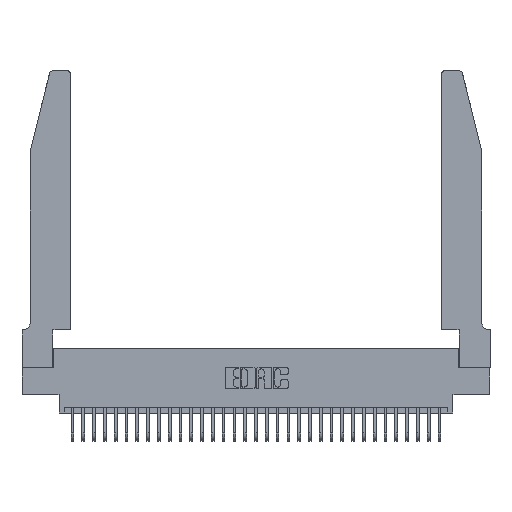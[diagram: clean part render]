
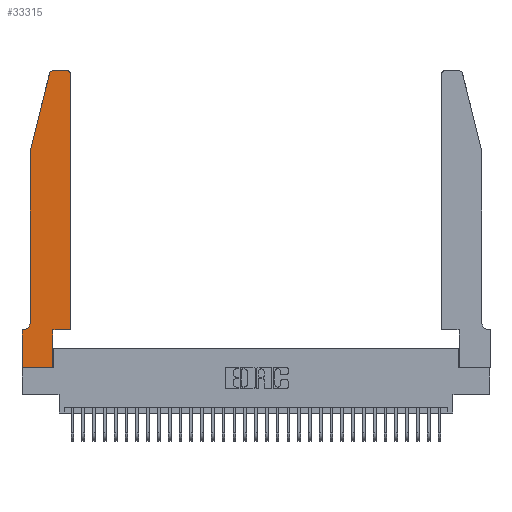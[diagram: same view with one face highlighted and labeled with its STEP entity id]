
A CAD part, top view. The second image highlights one B-rep face of the part: STEP entity #33315.
In plain terms, the highlighted planar face has unit normal (0, 0, 1).
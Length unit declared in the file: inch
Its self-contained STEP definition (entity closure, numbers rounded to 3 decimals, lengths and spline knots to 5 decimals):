
#8 = DIRECTION ( 'NONE',  ( 0., -1., 0. ) ) ;
#119 = ORIENTED_EDGE ( 'NONE', *, *, #659, .T. ) ;
#212 = VERTEX_POINT ( 'NONE', #12175 ) ;
#542 = DIRECTION ( 'NONE',  ( 0., 0., 1. ) ) ;
#655 = ORIENTED_EDGE ( 'NONE', *, *, #15621, .T. ) ;
#659 = EDGE_CURVE ( 'NONE', #1871, #23552, #33301, .T. ) ;
#753 = EDGE_CURVE ( 'NONE', #24900, #1871, #30790, .T. ) ;
#1272 = DIRECTION ( 'NONE',  ( -1., 0., 0. ) ) ;
#1370 = LINE ( 'NONE', #25315, #15069 ) ;
#1801 = VECTOR ( 'NONE', #9532, 39.37008 ) ;
#1871 = VERTEX_POINT ( 'NONE', #30890 ) ;
#2360 = CARTESIAN_POINT ( 'NONE',  ( 0.0755, 0.35, 0.37 ) ) ;
#2687 = CARTESIAN_POINT ( 'NONE',  ( 0.2865, 0., 0.37 ) ) ;
#3427 = LINE ( 'NONE', #26618, #30490 ) ;
#3617 = DIRECTION ( 'NONE',  ( 0., -1., 0. ) ) ;
#3751 = CARTESIAN_POINT ( 'NONE',  ( 0.4505, 2.72, 0.37 ) ) ;
#3753 = VECTOR ( 'NONE', #34737, 39.37008 ) ;
#3909 = ORIENTED_EDGE ( 'NONE', *, *, #30183, .T. ) ;
#4057 = CARTESIAN_POINT ( 'NONE',  ( 0.4205, 2.75, 0.37 ) ) ;
#4655 = CARTESIAN_POINT ( 'NONE',  ( 0.4505, 0.35, 0.37 ) ) ;
#5105 = EDGE_CURVE ( 'NONE', #23552, #212, #1370, .T. ) ;
#5524 = CARTESIAN_POINT ( 'NONE',  ( 0.0755, 2., 0.37 ) ) ;
#5705 = VERTEX_POINT ( 'NONE', #4057 ) ;
#6352 = FACE_OUTER_BOUND ( 'NONE', #27457, .T. ) ;
#7717 = CARTESIAN_POINT ( 'NONE',  ( 0., 0.35, 0.37 ) ) ;
#7741 = VECTOR ( 'NONE', #8, 39.37008 ) ;
#8313 = AXIS2_PLACEMENT_3D ( 'NONE', #29097, #13068, #31782 ) ;
#8574 = ORIENTED_EDGE ( 'NONE', *, *, #5105, .T. ) ;
#8948 = DIRECTION ( 'NONE',  ( 0., 1., 0. ) ) ;
#9012 = VERTEX_POINT ( 'NONE', #3751 ) ;
#9139 = ORIENTED_EDGE ( 'NONE', *, *, #31500, .T. ) ;
#9330 = VECTOR ( 'NONE', #26651, 39.37008 ) ;
#9532 = DIRECTION ( 'NONE',  ( 1., 0., 0. ) ) ;
#9984 = EDGE_CURVE ( 'NONE', #9012, #5705, #33779, .T. ) ;
#10199 = LINE ( 'NONE', #34577, #9330 ) ;
#12175 = CARTESIAN_POINT ( 'NONE',  ( 0., 0., 0.37 ) ) ;
#13068 = DIRECTION ( 'NONE',  ( 0., 0., 1. ) ) ;
#13121 = VECTOR ( 'NONE', #1272, 39.37008 ) ;
#14242 = DIRECTION ( 'NONE',  ( 0., 0., 1. ) ) ;
#14468 = CARTESIAN_POINT ( 'NONE',  ( 0.4505, 0.35, 0.37 ) ) ;
#14920 = VERTEX_POINT ( 'NONE', #14468 ) ;
#14981 = ORIENTED_EDGE ( 'NONE', *, *, #33085, .T. ) ;
#15069 = VECTOR ( 'NONE', #3617, 39.37008 ) ;
#15338 = VERTEX_POINT ( 'NONE', #32464 ) ;
#15621 = EDGE_CURVE ( 'NONE', #23240, #14920, #16352, .T. ) ;
#15879 = LINE ( 'NONE', #5524, #7741 ) ;
#16009 = CARTESIAN_POINT ( 'NONE',  ( 0.0755, 2., 0.37 ) ) ;
#16352 = LINE ( 'NONE', #20332, #1801 ) ;
#16680 = EDGE_CURVE ( 'NONE', #15338, #32474, #18363, .T. ) ;
#16897 = CARTESIAN_POINT ( 'NONE',  ( 0., 0.35, 0.37 ) ) ;
#17212 = CARTESIAN_POINT ( 'NONE',  ( 0.0755, 0.42, 0.37 ) ) ;
#17612 = CARTESIAN_POINT ( 'NONE',  ( 0.2605, 2.75, 0.37 ) ) ;
#18345 = ORIENTED_EDGE ( 'NONE', *, *, #32614, .T. ) ;
#18363 = CIRCLE ( 'NONE', #27455, 0.03 ) ;
#18371 = VERTEX_POINT ( 'NONE', #16009 ) ;
#18676 = CARTESIAN_POINT ( 'NONE',  ( 0.0055, 0.42, 0.37 ) ) ;
#18969 = ORIENTED_EDGE ( 'NONE', *, *, #26403, .T. ) ;
#19025 = AXIS2_PLACEMENT_3D ( 'NONE', #16897, #542, #19618 ) ;
#19618 = DIRECTION ( 'NONE',  ( 1., 0., 0. ) ) ;
#20332 = CARTESIAN_POINT ( 'NONE',  ( 0.4505, 0.35, 0.37 ) ) ;
#21391 = VERTEX_POINT ( 'NONE', #2687 ) ;
#22891 = CARTESIAN_POINT ( 'NONE',  ( 0.2865, 0.35, 0.37 ) ) ;
#23240 = VERTEX_POINT ( 'NONE', #22891 ) ;
#23552 = VERTEX_POINT ( 'NONE', #7717 ) ;
#23884 = CARTESIAN_POINT ( 'NONE',  ( 0.25487, 2.72718, 0.37 ) ) ;
#24280 = ORIENTED_EDGE ( 'NONE', *, *, #753, .T. ) ;
#24900 = VERTEX_POINT ( 'NONE', #17212 ) ;
#25315 = CARTESIAN_POINT ( 'NONE',  ( 0., 0., 0.37 ) ) ;
#26403 = EDGE_CURVE ( 'NONE', #32474, #18371, #3427, .T. ) ;
#26618 = CARTESIAN_POINT ( 'NONE',  ( 0.0755, 2., 0.37 ) ) ;
#26624 = ORIENTED_EDGE ( 'NONE', *, *, #16680, .T. ) ;
#26651 = DIRECTION ( 'NONE',  ( 1., 0., 0. ) ) ;
#26676 = LINE ( 'NONE', #4655, #32932 ) ;
#27455 = AXIS2_PLACEMENT_3D ( 'NONE', #30277, #14242, #32953 ) ;
#27457 = EDGE_LOOP ( 'NONE', ( #3909, #26624, #18969, #18345, #24280, #119, #8574, #28551, #9139, #655, #14981, #28724 ) ) ;
#27968 = EDGE_CURVE ( 'NONE', #212, #21391, #10199, .T. ) ;
#28551 = ORIENTED_EDGE ( 'NONE', *, *, #27968, .T. ) ;
#28724 = ORIENTED_EDGE ( 'NONE', *, *, #9984, .T. ) ;
#28934 = VECTOR ( 'NONE', #8948, 39.37008 ) ;
#28935 = AXIS2_PLACEMENT_3D ( 'NONE', #18676, #29413, #33131 ) ;
#28974 = DIRECTION ( 'NONE',  ( 0., 1., 0. ) ) ;
#29097 = CARTESIAN_POINT ( 'NONE',  ( 0.4205, 2.72, 0.37 ) ) ;
#29281 = DIRECTION ( 'NONE',  ( -0.239, -0.971, 0. ) ) ;
#29413 = DIRECTION ( 'NONE',  ( 0., 0., -1. ) ) ;
#29764 = LINE ( 'NONE', #30479, #28934 ) ;
#30183 = EDGE_CURVE ( 'NONE', #5705, #15338, #32788, .T. ) ;
#30277 = CARTESIAN_POINT ( 'NONE',  ( 0.284, 2.72, 0.37 ) ) ;
#30479 = CARTESIAN_POINT ( 'NONE',  ( 0.2865, 0.35, 0.37 ) ) ;
#30490 = VECTOR ( 'NONE', #29281, 39.37008 ) ;
#30790 = CIRCLE ( 'NONE', #28935, 0.07 ) ;
#30890 = CARTESIAN_POINT ( 'NONE',  ( 0.0055, 0.35, 0.37 ) ) ;
#31500 = EDGE_CURVE ( 'NONE', #21391, #23240, #29764, .T. ) ;
#31782 = DIRECTION ( 'NONE',  ( 1., 0., 0. ) ) ;
#32464 = CARTESIAN_POINT ( 'NONE',  ( 0.284, 2.75, 0.37 ) ) ;
#32474 = VERTEX_POINT ( 'NONE', #23884 ) ;
#32614 = EDGE_CURVE ( 'NONE', #18371, #24900, #15879, .T. ) ;
#32788 = LINE ( 'NONE', #17612, #13121 ) ;
#32912 = PLANE ( 'NONE',  #19025 ) ;
#32932 = VECTOR ( 'NONE', #28974, 39.37008 ) ;
#32953 = DIRECTION ( 'NONE',  ( 1., 0., 0. ) ) ;
#33085 = EDGE_CURVE ( 'NONE', #14920, #9012, #26676, .T. ) ;
#33131 = DIRECTION ( 'NONE',  ( -1., 0., 0. ) ) ;
#33301 = LINE ( 'NONE', #2360, #3753 ) ;
#33315 = ADVANCED_FACE ( 'NONE', ( #6352 ), #32912, .T. ) ;
#33779 = CIRCLE ( 'NONE', #8313, 0.03 ) ;
#34577 = CARTESIAN_POINT ( 'NONE',  ( 0., 0., 0.37 ) ) ;
#34737 = DIRECTION ( 'NONE',  ( -1., 0., 0. ) ) ;
